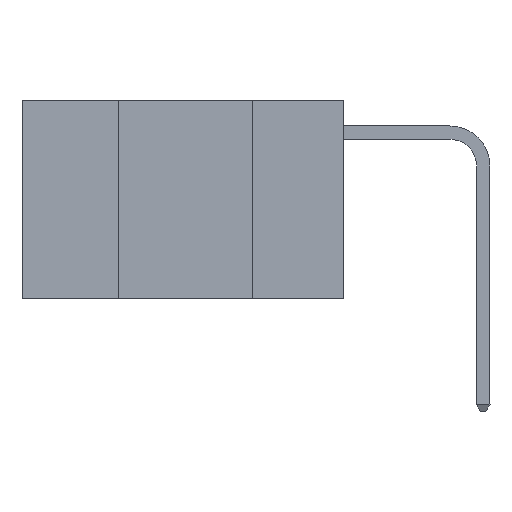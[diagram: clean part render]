
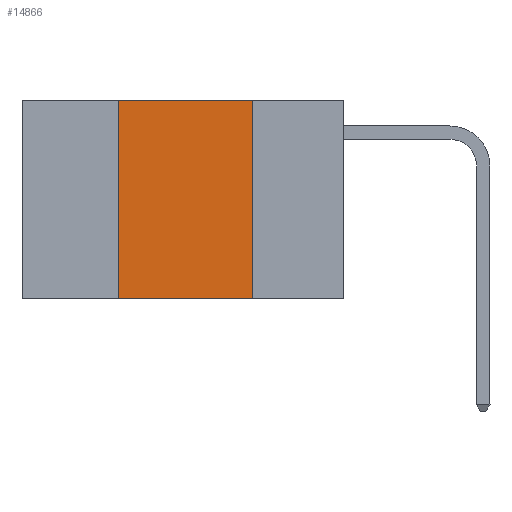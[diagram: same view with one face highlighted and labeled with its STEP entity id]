
A CAD part, left-side view. The second image highlights one B-rep face of the part: STEP entity #14866.
In plain terms, the highlighted planar face has unit normal (-1, 0, 0).
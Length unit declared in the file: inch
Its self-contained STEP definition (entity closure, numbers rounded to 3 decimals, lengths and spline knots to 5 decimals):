
#294 = LINE ( 'NONE', #771, #7181 ) ;
#771 = CARTESIAN_POINT ( 'NONE',  ( 0., 0.17, 0. ) ) ;
#1124 = VECTOR ( 'NONE', #11568, 39.37008 ) ;
#1138 = EDGE_CURVE ( 'NONE', #8588, #7575, #7698, .T. ) ;
#2449 = EDGE_CURVE ( 'NONE', #7575, #5618, #294, .T. ) ;
#2837 = CARTESIAN_POINT ( 'NONE',  ( 0., 0.6, -0.37 ) ) ;
#3092 = VECTOR ( 'NONE', #5990, 39.37008 ) ;
#3274 = PLANE ( 'NONE',  #7449 ) ;
#3345 = CARTESIAN_POINT ( 'NONE',  ( 0., 0.6, 0. ) ) ;
#3794 = CARTESIAN_POINT ( 'NONE',  ( 0., 0.42, -0.37 ) ) ;
#3878 = VECTOR ( 'NONE', #6740, 39.37008 ) ;
#4835 = DIRECTION ( 'NONE',  ( 0., 0., -1. ) ) ;
#5618 = VERTEX_POINT ( 'NONE', #9915 ) ;
#5990 = DIRECTION ( 'NONE',  ( 0., 0., 1. ) ) ;
#6740 = DIRECTION ( 'NONE',  ( 0., -1., 0. ) ) ;
#7181 = VECTOR ( 'NONE', #15198, 39.37008 ) ;
#7404 = LINE ( 'NONE', #10319, #3092 ) ;
#7449 = AXIS2_PLACEMENT_3D ( 'NONE', #3345, #13496, #4835 ) ;
#7575 = VERTEX_POINT ( 'NONE', #13618 ) ;
#7698 = LINE ( 'NONE', #16742, #3878 ) ;
#8588 = VERTEX_POINT ( 'NONE', #14325 ) ;
#8972 = ORIENTED_EDGE ( 'NONE', *, *, #1138, .F. ) ;
#9028 = ORIENTED_EDGE ( 'NONE', *, *, #13424, .T. ) ;
#9052 = ORIENTED_EDGE ( 'NONE', *, *, #9291, .F. ) ;
#9291 = EDGE_CURVE ( 'NONE', #13711, #8588, #7404, .T. ) ;
#9915 = CARTESIAN_POINT ( 'NONE',  ( 0., 0.17, -0.37 ) ) ;
#9994 = ORIENTED_EDGE ( 'NONE', *, *, #2449, .F. ) ;
#10319 = CARTESIAN_POINT ( 'NONE',  ( 0., 0.42, 0. ) ) ;
#11568 = DIRECTION ( 'NONE',  ( 0., -1., 0. ) ) ;
#13424 = EDGE_CURVE ( 'NONE', #13711, #5618, #15867, .T. ) ;
#13496 = DIRECTION ( 'NONE',  ( 1., 0., 0. ) ) ;
#13618 = CARTESIAN_POINT ( 'NONE',  ( 0., 0.17, 0. ) ) ;
#13711 = VERTEX_POINT ( 'NONE', #3794 ) ;
#13905 = FACE_OUTER_BOUND ( 'NONE', #15083, .T. ) ;
#14325 = CARTESIAN_POINT ( 'NONE',  ( 0., 0.42, 0. ) ) ;
#14866 = ADVANCED_FACE ( 'NONE', ( #13905 ), #3274, .F. ) ;
#15083 = EDGE_LOOP ( 'NONE', ( #9994, #8972, #9052, #9028 ) ) ;
#15198 = DIRECTION ( 'NONE',  ( 0., 0., -1. ) ) ;
#15867 = LINE ( 'NONE', #2837, #1124 ) ;
#16742 = CARTESIAN_POINT ( 'NONE',  ( 0., 0.6, 0. ) ) ;
